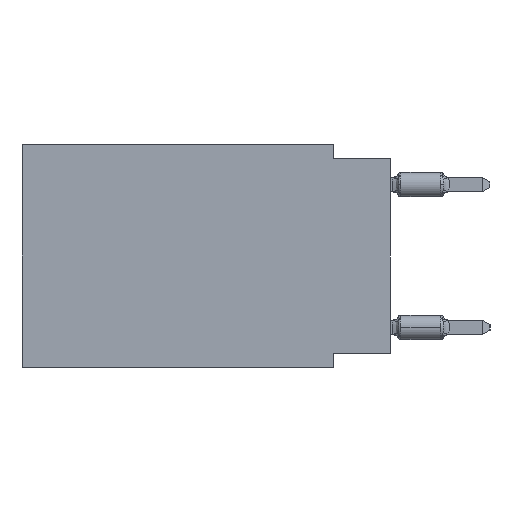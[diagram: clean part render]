
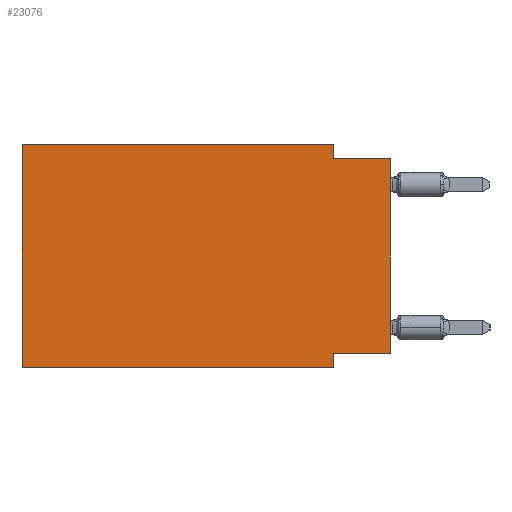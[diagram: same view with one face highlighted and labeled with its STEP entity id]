
A CAD part, left-side view. The second image highlights one B-rep face of the part: STEP entity #23076.
In plain terms, the highlighted planar face has unit normal (-1, 0, 0).
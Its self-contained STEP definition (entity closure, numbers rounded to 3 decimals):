
#88 = CARTESIAN_POINT ( 'NONE',  ( 0., 16.383, 0. ) ) ;
#111 = VECTOR ( 'NONE', #2254, 1000. ) ;
#218 = DIRECTION ( 'NONE',  ( 1., 0., 0. ) ) ;
#607 = AXIS2_PLACEMENT_3D ( 'NONE', #88, #218, #7556 ) ;
#1730 = CARTESIAN_POINT ( 'NONE',  ( 0., 2.54, 0. ) ) ;
#2254 = DIRECTION ( 'NONE',  ( 0., -1., 0. ) ) ;
#2404 = LINE ( 'NONE', #17214, #19470 ) ;
#2600 = VERTEX_POINT ( 'NONE', #15875 ) ;
#3185 = EDGE_CURVE ( 'NONE', #18389, #9651, #20370, .T. ) ;
#3248 = LINE ( 'NONE', #20138, #5528 ) ;
#3602 = DIRECTION ( 'NONE',  ( 0., 0., -1. ) ) ;
#3645 = FACE_OUTER_BOUND ( 'NONE', #18738, .T. ) ;
#3811 = ORIENTED_EDGE ( 'NONE', *, *, #12766, .F. ) ;
#3898 = ORIENTED_EDGE ( 'NONE', *, *, #3185, .F. ) ;
#5528 = VECTOR ( 'NONE', #18054, 1000. ) ;
#5908 = CARTESIAN_POINT ( 'NONE',  ( 0., 0., -0.635 ) ) ;
#6209 = CARTESIAN_POINT ( 'NONE',  ( 0., 0., -9.271 ) ) ;
#7013 = CARTESIAN_POINT ( 'NONE',  ( 0., 16.383, 0. ) ) ;
#7556 = DIRECTION ( 'NONE',  ( 0., 0., -1. ) ) ;
#7879 = LINE ( 'NONE', #11058, #111 ) ;
#8291 = VERTEX_POINT ( 'NONE', #7013 ) ;
#8452 = CARTESIAN_POINT ( 'NONE',  ( 0., 16.383, 0. ) ) ;
#9070 = CARTESIAN_POINT ( 'NONE',  ( 0., 2.54, -9.271 ) ) ;
#9651 = VERTEX_POINT ( 'NONE', #24180 ) ;
#9935 = VECTOR ( 'NONE', #17391, 1000. ) ;
#10069 = ORIENTED_EDGE ( 'NONE', *, *, #13871, .T. ) ;
#10166 = LINE ( 'NONE', #22777, #16880 ) ;
#10940 = LINE ( 'NONE', #12529, #23575 ) ;
#11058 = CARTESIAN_POINT ( 'NONE',  ( 0., 0., -0.635 ) ) ;
#11478 = PLANE ( 'NONE',  #607 ) ;
#11642 = VERTEX_POINT ( 'NONE', #5908 ) ;
#11725 = VERTEX_POINT ( 'NONE', #16678 ) ;
#12529 = CARTESIAN_POINT ( 'NONE',  ( 0., 16.383, -9.906 ) ) ;
#12766 = EDGE_CURVE ( 'NONE', #11725, #11642, #7879, .T. ) ;
#13837 = DIRECTION ( 'NONE',  ( 0., 1., 0. ) ) ;
#13871 = EDGE_CURVE ( 'NONE', #2600, #9651, #10940, .T. ) ;
#14534 = EDGE_CURVE ( 'NONE', #2600, #8291, #15549, .T. ) ;
#15172 = ORIENTED_EDGE ( 'NONE', *, *, #14534, .F. ) ;
#15500 = DIRECTION ( 'NONE',  ( 0., 0., 1. ) ) ;
#15549 = LINE ( 'NONE', #8452, #9935 ) ;
#15875 = CARTESIAN_POINT ( 'NONE',  ( 0., 16.383, -9.906 ) ) ;
#16212 = EDGE_CURVE ( 'NONE', #18403, #11725, #3248, .T. ) ;
#16568 = DIRECTION ( 'NONE',  ( 0., -1., 0. ) ) ;
#16678 = CARTESIAN_POINT ( 'NONE',  ( 0., 2.54, -0.635 ) ) ;
#16880 = VECTOR ( 'NONE', #13837, 1000. ) ;
#16958 = EDGE_CURVE ( 'NONE', #21902, #18389, #10166, .T. ) ;
#17214 = CARTESIAN_POINT ( 'NONE',  ( 0., 0., 0. ) ) ;
#17391 = DIRECTION ( 'NONE',  ( 0., 0., 1. ) ) ;
#17765 = ORIENTED_EDGE ( 'NONE', *, *, #16212, .F. ) ;
#17990 = ORIENTED_EDGE ( 'NONE', *, *, #16958, .F. ) ;
#18054 = DIRECTION ( 'NONE',  ( 0., 0., -1. ) ) ;
#18389 = VERTEX_POINT ( 'NONE', #9070 ) ;
#18403 = VERTEX_POINT ( 'NONE', #1730 ) ;
#18738 = EDGE_LOOP ( 'NONE', ( #22141, #3811, #17765, #20502, #15172, #10069, #3898, #17990 ) ) ;
#19444 = DIRECTION ( 'NONE',  ( 0., -1., 0. ) ) ;
#19470 = VECTOR ( 'NONE', #15500, 1000. ) ;
#20138 = CARTESIAN_POINT ( 'NONE',  ( 0., 2.54, 0. ) ) ;
#20268 = EDGE_CURVE ( 'NONE', #8291, #18403, #22865, .T. ) ;
#20370 = LINE ( 'NONE', #20492, #23268 ) ;
#20492 = CARTESIAN_POINT ( 'NONE',  ( 0., 2.54, -9.906 ) ) ;
#20502 = ORIENTED_EDGE ( 'NONE', *, *, #20268, .F. ) ;
#21750 = VECTOR ( 'NONE', #19444, 1000. ) ;
#21902 = VERTEX_POINT ( 'NONE', #6209 ) ;
#21967 = EDGE_CURVE ( 'NONE', #21902, #11642, #2404, .T. ) ;
#22141 = ORIENTED_EDGE ( 'NONE', *, *, #21967, .T. ) ;
#22777 = CARTESIAN_POINT ( 'NONE',  ( 0., 0., -9.271 ) ) ;
#22865 = LINE ( 'NONE', #22988, #21750 ) ;
#22988 = CARTESIAN_POINT ( 'NONE',  ( 0., 16.383, 0. ) ) ;
#23076 = ADVANCED_FACE ( 'NONE', ( #3645 ), #11478, .F. ) ;
#23268 = VECTOR ( 'NONE', #3602, 1000. ) ;
#23575 = VECTOR ( 'NONE', #16568, 1000. ) ;
#24180 = CARTESIAN_POINT ( 'NONE',  ( 0., 2.54, -9.906 ) ) ;
